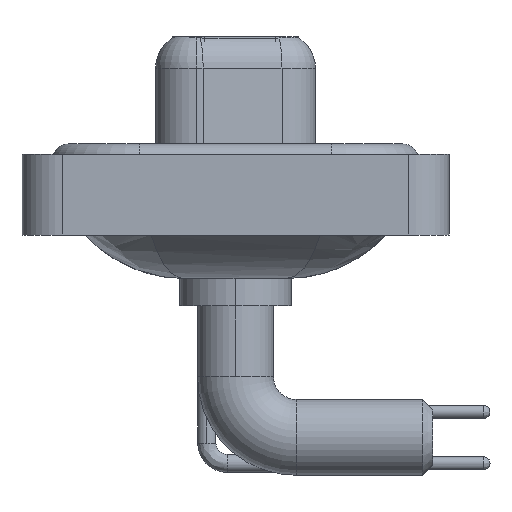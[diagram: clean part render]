
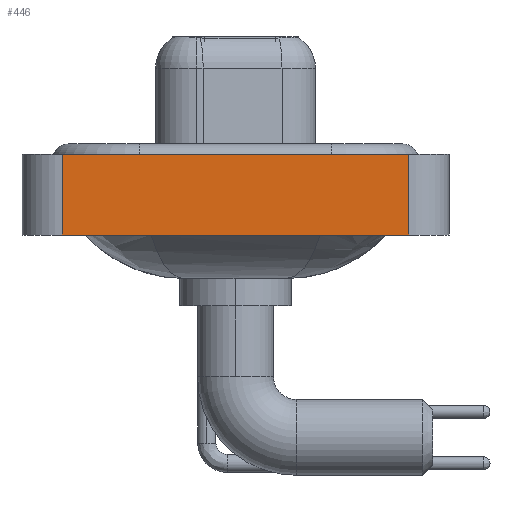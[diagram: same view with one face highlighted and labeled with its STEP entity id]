
A CAD part, left-side view. The second image highlights one B-rep face of the part: STEP entity #446.
In plain terms, the highlighted planar face has unit normal (-1, 0, 0).
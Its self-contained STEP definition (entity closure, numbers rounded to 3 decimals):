
#201 = EDGE_CURVE ( 'NONE', #11073, #19928, #10575, .T. ) ;
#446 = ADVANCED_FACE ( 'NONE', ( #8569 ), #19878, .T. ) ;
#982 = VECTOR ( 'NONE', #16588, 1000. ) ;
#1291 = LINE ( 'NONE', #15799, #12522 ) ;
#3296 = EDGE_CURVE ( 'NONE', #9818, #19928, #16482, .T. ) ;
#5159 = VECTOR ( 'NONE', #16955, 1000. ) ;
#6011 = VERTEX_POINT ( 'NONE', #9067 ) ;
#6219 = ORIENTED_EDGE ( 'NONE', *, *, #3296, .T. ) ;
#7932 = EDGE_CURVE ( 'NONE', #6011, #11073, #1291, .T. ) ;
#8569 = FACE_OUTER_BOUND ( 'NONE', #20409, .T. ) ;
#8791 = EDGE_CURVE ( 'NONE', #6011, #9818, #12031, .T. ) ;
#8819 = CARTESIAN_POINT ( 'NONE',  ( -7.35, -8.55, 0.4 ) ) ;
#9067 = CARTESIAN_POINT ( 'NONE',  ( -7.35, 8.55, -3.6 ) ) ;
#9818 = VERTEX_POINT ( 'NONE', #20505 ) ;
#10416 = ORIENTED_EDGE ( 'NONE', *, *, #201, .F. ) ;
#10575 = LINE ( 'NONE', #13682, #5159 ) ;
#10808 = DIRECTION ( 'NONE',  ( 0., 0., 1. ) ) ;
#11073 = VERTEX_POINT ( 'NONE', #19438 ) ;
#11626 = CARTESIAN_POINT ( 'NONE',  ( -7.35, -8.55, -3.6 ) ) ;
#11823 = DIRECTION ( 'NONE',  ( 0., -1., 0. ) ) ;
#12031 = LINE ( 'NONE', #19986, #12534 ) ;
#12522 = VECTOR ( 'NONE', #10808, 1000. ) ;
#12534 = VECTOR ( 'NONE', #11823, 1000. ) ;
#13337 = DIRECTION ( 'NONE',  ( -1., 0., 0. ) ) ;
#13432 = DIRECTION ( 'NONE',  ( 0., 0., 1. ) ) ;
#13682 = CARTESIAN_POINT ( 'NONE',  ( -7.35, -8.55, 0.4 ) ) ;
#15019 = CARTESIAN_POINT ( 'NONE',  ( -7.35, -8.55, -3.6 ) ) ;
#15799 = CARTESIAN_POINT ( 'NONE',  ( -7.35, 8.55, -3.6 ) ) ;
#15992 = AXIS2_PLACEMENT_3D ( 'NONE', #11626, #13337, #13432 ) ;
#16386 = ORIENTED_EDGE ( 'NONE', *, *, #7932, .F. ) ;
#16482 = LINE ( 'NONE', #15019, #982 ) ;
#16588 = DIRECTION ( 'NONE',  ( 0., 0., 1. ) ) ;
#16927 = ORIENTED_EDGE ( 'NONE', *, *, #8791, .T. ) ;
#16955 = DIRECTION ( 'NONE',  ( 0., -1., 0. ) ) ;
#19438 = CARTESIAN_POINT ( 'NONE',  ( -7.35, 8.55, 0.4 ) ) ;
#19878 = PLANE ( 'NONE',  #15992 ) ;
#19928 = VERTEX_POINT ( 'NONE', #8819 ) ;
#19986 = CARTESIAN_POINT ( 'NONE',  ( -7.35, -8.55, -3.6 ) ) ;
#20409 = EDGE_LOOP ( 'NONE', ( #6219, #10416, #16386, #16927 ) ) ;
#20505 = CARTESIAN_POINT ( 'NONE',  ( -7.35, -8.55, -3.6 ) ) ;
